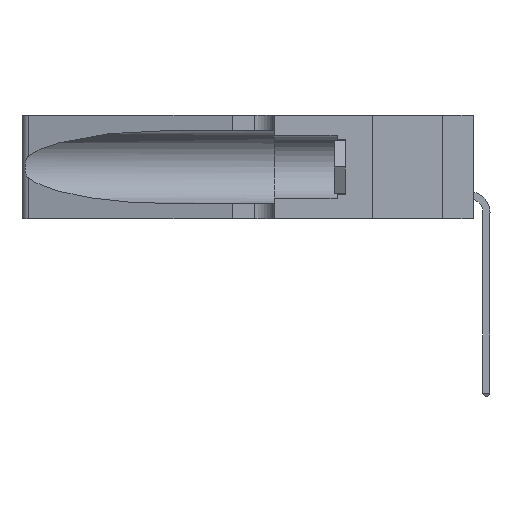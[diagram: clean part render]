
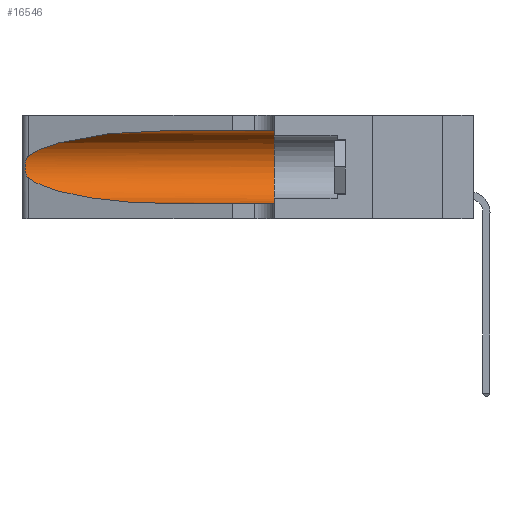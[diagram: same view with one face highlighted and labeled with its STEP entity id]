
A CAD part, left-side view. The second image highlights one B-rep face of the part: STEP entity #16546.
In plain terms, the highlighted cylindrical face has radius 3.308 mm (diameter 6.617 mm), a partial arc.
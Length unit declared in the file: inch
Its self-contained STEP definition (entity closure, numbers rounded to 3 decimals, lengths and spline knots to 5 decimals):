
#331 = LINE ( 'NONE', #4077, #2863 ) ;
#462 = CARTESIAN_POINT ( 'NONE',  ( 0.18966, 0.96281, 0.05475 ) ) ;
#672 = VERTEX_POINT ( 'NONE', #4633 ) ;
#678 = DIRECTION ( 'NONE',  ( 0., -1., 0. ) ) ;
#1231 = EDGE_CURVE ( 'NONE', #13723, #6613, #331, .T. ) ;
#1395 = CARTESIAN_POINT ( 'NONE',  ( 0.25856, 1.23593, 0.16098 ) ) ;
#1681 = B_SPLINE_CURVE_WITH_KNOTS ( 'NONE', 3,
 ( #13409, #14732, #11837, #17160, #6773, #7920, #15867, #16062, #8087, #1395, #10793, #10559, #2512, #11891 ),
 .UNSPECIFIED., .F., .F.,
 ( 4, 2, 2, 2, 2, 2, 4 ),
 ( 0., 0.00027, 0.00053, 0.00107, 0.0016, 0.00187, 0.00214 ),
 .UNSPECIFIED. ) ;
#2424 = FACE_OUTER_BOUND ( 'NONE', #11672, .T. ) ;
#2512 = CARTESIAN_POINT ( 'NONE',  ( 0.25555, 1.22993, 0.14849 ) ) ;
#2664 =( BOUNDED_CURVE ( )  B_SPLINE_CURVE ( 3, ( #5729, #5670, #462, #15148 ),
 .UNSPECIFIED., .F., .T. ) 
 B_SPLINE_CURVE_WITH_KNOTS ( ( 4, 4 ),
 ( 3.44316, 4.71239 ),
 .UNSPECIFIED. ) 
 CURVE ( )  GEOMETRIC_REPRESENTATION_ITEM ( )  RATIONAL_B_SPLINE_CURVE ( ( 1., 0.87, 0.87, 1. ) ) 
 REPRESENTATION_ITEM ( '' )  );
#2863 = VECTOR ( 'NONE', #4875, 39.37008 ) ;
#3337 = CARTESIAN_POINT ( 'NONE',  ( 0.1305, 1.61858, 0.05475 ) ) ;
#3810 = EDGE_CURVE ( 'NONE', #6613, #17096, #14078, .T. ) ;
#3869 = CARTESIAN_POINT ( 'NONE',  ( 0.1305, 0.72297, 0.31525 ) ) ;
#3912 = EDGE_CURVE ( 'NONE', #9775, #17096, #7837, .T. ) ;
#4077 = CARTESIAN_POINT ( 'NONE',  ( 0.1305, 1.61858, 0.31525 ) ) ;
#4633 = CARTESIAN_POINT ( 'NONE',  ( 0.25487, 1.22718, 0.14631 ) ) ;
#4875 = DIRECTION ( 'NONE',  ( 0., -1., 0. ) ) ;
#5410 = CARTESIAN_POINT ( 'NONE',  ( 0.18966, 0.96281, 0.31525 ) ) ;
#5670 = CARTESIAN_POINT ( 'NONE',  ( 0.2373, 1.15595, 0.08982 ) ) ;
#5729 = CARTESIAN_POINT ( 'NONE',  ( 0.25487, 1.22718, 0.14631 ) ) ;
#5762 = CARTESIAN_POINT ( 'NONE',  ( 0.1305, 0.35, 0.05475 ) ) ;
#6003 = CARTESIAN_POINT ( 'NONE',  ( 0.1305, 1.61858, 0.185 ) ) ;
#6049 = DIRECTION ( 'NONE',  ( 0., 1., 0. ) ) ;
#6110 = DIRECTION ( 'NONE',  ( 0., 0., -1. ) ) ;
#6163 = DIRECTION ( 'NONE',  ( 0., 0., 1. ) ) ;
#6352 = ORIENTED_EDGE ( 'NONE', *, *, #16499, .T. ) ;
#6540 = ORIENTED_EDGE ( 'NONE', *, *, #16849, .T. ) ;
#6613 = VERTEX_POINT ( 'NONE', #9756 ) ;
#6773 = CARTESIAN_POINT ( 'NONE',  ( 0.25854, 1.2359, 0.20912 ) ) ;
#6831 = ORIENTED_EDGE ( 'NONE', *, *, #16803, .T. ) ;
#7321 = ORIENTED_EDGE ( 'NONE', *, *, #1231, .F. ) ;
#7404 = DIRECTION ( 'NONE',  ( 0., -1., 0. ) ) ;
#7837 = LINE ( 'NONE', #3337, #12411 ) ;
#7920 = CARTESIAN_POINT ( 'NONE',  ( 0.26018, 1.23835, 0.19895 ) ) ;
#8087 = CARTESIAN_POINT ( 'NONE',  ( 0.26017, 1.23833, 0.17102 ) ) ;
#8145 =( BOUNDED_CURVE ( )  B_SPLINE_CURVE ( 3, ( #3869, #5410, #9315, #13164 ),
 .UNSPECIFIED., .F., .T. ) 
 B_SPLINE_CURVE_WITH_KNOTS ( ( 4, 4 ),
 ( 1.5708, 2.84003 ),
 .UNSPECIFIED. ) 
 CURVE ( )  GEOMETRIC_REPRESENTATION_ITEM ( )  RATIONAL_B_SPLINE_CURVE ( ( 1., 0.87, 0.87, 1. ) ) 
 REPRESENTATION_ITEM ( '' )  );
#8425 = CARTESIAN_POINT ( 'NONE',  ( 0.1305, 0.72297, 0.05475 ) ) ;
#9150 = CYLINDRICAL_SURFACE ( 'NONE', #16686, 0.13025 ) ;
#9315 = CARTESIAN_POINT ( 'NONE',  ( 0.2373, 1.15595, 0.28018 ) ) ;
#9756 = CARTESIAN_POINT ( 'NONE',  ( 0.1305, 0.35, 0.31525 ) ) ;
#9775 = VERTEX_POINT ( 'NONE', #8425 ) ;
#9956 = CARTESIAN_POINT ( 'NONE',  ( 0.1305, 0.35, 0.185 ) ) ;
#10559 = CARTESIAN_POINT ( 'NONE',  ( 0.25639, 1.23186, 0.15144 ) ) ;
#10793 = CARTESIAN_POINT ( 'NONE',  ( 0.25789, 1.23486, 0.15765 ) ) ;
#10832 = VERTEX_POINT ( 'NONE', #13475 ) ;
#11085 = AXIS2_PLACEMENT_3D ( 'NONE', #9956, #6049, #6163 ) ;
#11672 = EDGE_LOOP ( 'NONE', ( #6831, #6540, #6352, #12638, #14790, #7321 ) ) ;
#11837 = CARTESIAN_POINT ( 'NONE',  ( 0.25639, 1.23184, 0.21858 ) ) ;
#11891 = CARTESIAN_POINT ( 'NONE',  ( 0.25487, 1.22718, 0.14631 ) ) ;
#12411 = VECTOR ( 'NONE', #678, 39.37008 ) ;
#12638 = ORIENTED_EDGE ( 'NONE', *, *, #3912, .T. ) ;
#13164 = CARTESIAN_POINT ( 'NONE',  ( 0.25487, 1.22718, 0.22369 ) ) ;
#13409 = CARTESIAN_POINT ( 'NONE',  ( 0.25487, 1.22718, 0.22369 ) ) ;
#13475 = CARTESIAN_POINT ( 'NONE',  ( 0.25487, 1.22718, 0.22369 ) ) ;
#13723 = VERTEX_POINT ( 'NONE', #16492 ) ;
#14078 = CIRCLE ( 'NONE', #11085, 0.13025 ) ;
#14732 = CARTESIAN_POINT ( 'NONE',  ( 0.25555, 1.22994, 0.2215 ) ) ;
#14790 = ORIENTED_EDGE ( 'NONE', *, *, #3810, .F. ) ;
#15148 = CARTESIAN_POINT ( 'NONE',  ( 0.1305, 0.72297, 0.05475 ) ) ;
#15867 = CARTESIAN_POINT ( 'NONE',  ( 0.26075, 1.23896, 0.19203 ) ) ;
#16062 = CARTESIAN_POINT ( 'NONE',  ( 0.26075, 1.23896, 0.178 ) ) ;
#16492 = CARTESIAN_POINT ( 'NONE',  ( 0.1305, 0.72297, 0.31525 ) ) ;
#16499 = EDGE_CURVE ( 'NONE', #672, #9775, #2664, .T. ) ;
#16546 = ADVANCED_FACE ( 'NONE', ( #2424 ), #9150, .F. ) ;
#16686 = AXIS2_PLACEMENT_3D ( 'NONE', #6003, #7404, #6110 ) ;
#16803 = EDGE_CURVE ( 'NONE', #13723, #10832, #8145, .T. ) ;
#16849 = EDGE_CURVE ( 'NONE', #10832, #672, #1681, .T. ) ;
#17096 = VERTEX_POINT ( 'NONE', #5762 ) ;
#17160 = CARTESIAN_POINT ( 'NONE',  ( 0.25787, 1.23484, 0.2124 ) ) ;
